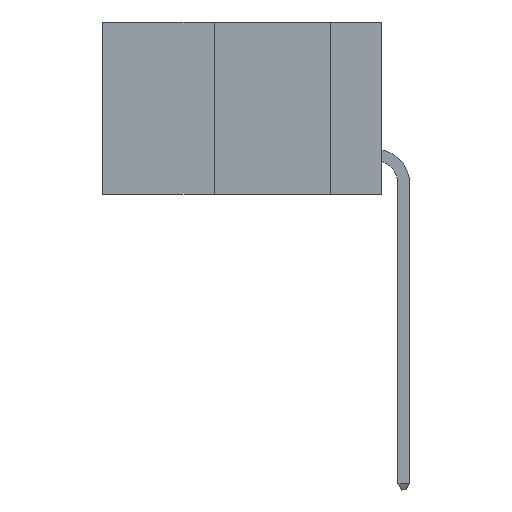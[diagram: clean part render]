
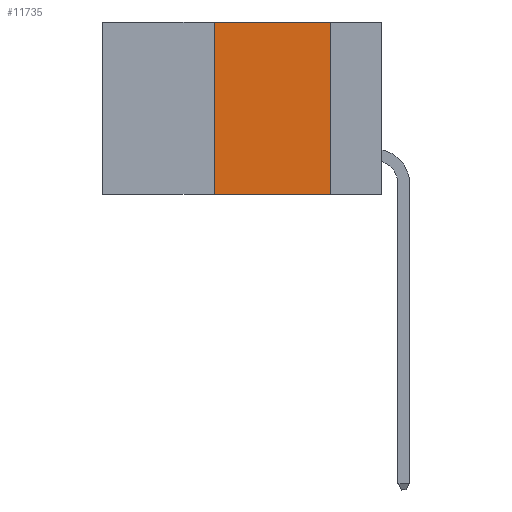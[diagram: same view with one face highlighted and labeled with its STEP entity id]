
A CAD part, left-side view. The second image highlights one B-rep face of the part: STEP entity #11735.
In plain terms, the highlighted planar face has unit normal (-1, 0, 0).
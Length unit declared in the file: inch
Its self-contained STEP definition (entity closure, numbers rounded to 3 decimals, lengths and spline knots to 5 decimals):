
#18 = CARTESIAN_POINT ( 'NONE',  ( 0., 0.36, -0.37 ) ) ;
#252 = CARTESIAN_POINT ( 'NONE',  ( 0., 0.6, 0. ) ) ;
#542 = LINE ( 'NONE', #23318, #11709 ) ;
#578 = VERTEX_POINT ( 'NONE', #9397 ) ;
#2061 = ORIENTED_EDGE ( 'NONE', *, *, #8744, .F. ) ;
#2335 = VERTEX_POINT ( 'NONE', #16946 ) ;
#3296 = PLANE ( 'NONE',  #4775 ) ;
#4775 = AXIS2_PLACEMENT_3D ( 'NONE', #15089, #23109, #5206 ) ;
#5206 = DIRECTION ( 'NONE',  ( 0., 0., -1. ) ) ;
#5249 = DIRECTION ( 'NONE',  ( 0., -1., 0. ) ) ;
#7980 = DIRECTION ( 'NONE',  ( 0., 0., -1. ) ) ;
#8744 = EDGE_CURVE ( 'NONE', #20353, #25542, #11855, .T. ) ;
#8746 = CARTESIAN_POINT ( 'NONE',  ( 0., 0.36, 0. ) ) ;
#9397 = CARTESIAN_POINT ( 'NONE',  ( 0., 0.11, -0.37 ) ) ;
#10404 = EDGE_LOOP ( 'NONE', ( #25177, #17877, #2061, #16746 ) ) ;
#11277 = EDGE_CURVE ( 'NONE', #20353, #578, #542, .T. ) ;
#11709 = VECTOR ( 'NONE', #5249, 39.37008 ) ;
#11735 = ADVANCED_FACE ( 'NONE', ( #12702 ), #3296, .F. ) ;
#11740 = CARTESIAN_POINT ( 'NONE',  ( 0., 0.36, 0. ) ) ;
#11855 = LINE ( 'NONE', #8746, #15267 ) ;
#12702 = FACE_OUTER_BOUND ( 'NONE', #10404, .T. ) ;
#15089 = CARTESIAN_POINT ( 'NONE',  ( 0., 0.6, 0. ) ) ;
#15267 = VECTOR ( 'NONE', #24531, 39.37008 ) ;
#16282 = VECTOR ( 'NONE', #17994, 39.37008 ) ;
#16746 = ORIENTED_EDGE ( 'NONE', *, *, #11277, .T. ) ;
#16946 = CARTESIAN_POINT ( 'NONE',  ( 0., 0.11, 0. ) ) ;
#17877 = ORIENTED_EDGE ( 'NONE', *, *, #17882, .F. ) ;
#17882 = EDGE_CURVE ( 'NONE', #25542, #2335, #23416, .T. ) ;
#17994 = DIRECTION ( 'NONE',  ( 0., -1., 0. ) ) ;
#19612 = VECTOR ( 'NONE', #7980, 39.37008 ) ;
#19649 = EDGE_CURVE ( 'NONE', #2335, #578, #22093, .T. ) ;
#20353 = VERTEX_POINT ( 'NONE', #18 ) ;
#22093 = LINE ( 'NONE', #23887, #19612 ) ;
#23109 = DIRECTION ( 'NONE',  ( 1., 0., 0. ) ) ;
#23318 = CARTESIAN_POINT ( 'NONE',  ( 0., 0.6, -0.37 ) ) ;
#23416 = LINE ( 'NONE', #252, #16282 ) ;
#23887 = CARTESIAN_POINT ( 'NONE',  ( 0., 0.11, 0. ) ) ;
#24531 = DIRECTION ( 'NONE',  ( 0., 0., 1. ) ) ;
#25177 = ORIENTED_EDGE ( 'NONE', *, *, #19649, .F. ) ;
#25542 = VERTEX_POINT ( 'NONE', #11740 ) ;
